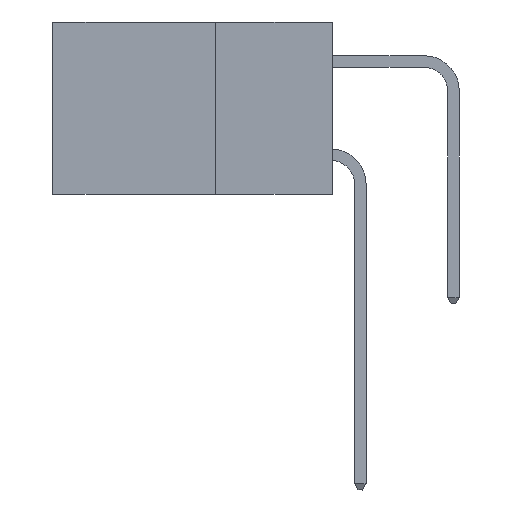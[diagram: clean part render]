
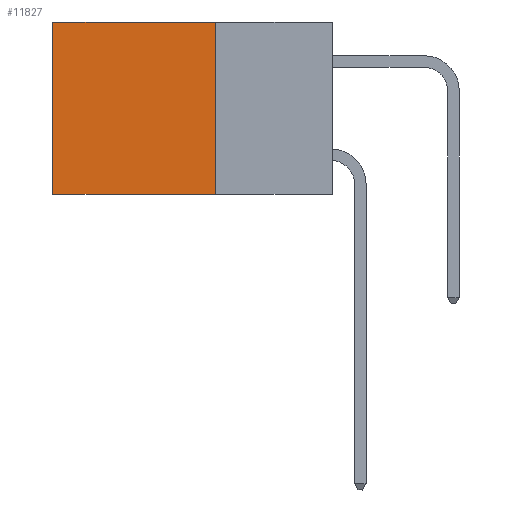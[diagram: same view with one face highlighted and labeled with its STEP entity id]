
A CAD part, left-side view. The second image highlights one B-rep face of the part: STEP entity #11827.
In plain terms, the highlighted planar face has unit normal (-1, 0, 0).
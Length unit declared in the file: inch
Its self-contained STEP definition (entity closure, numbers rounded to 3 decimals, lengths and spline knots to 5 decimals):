
#1057 = LINE ( 'NONE', #18911, #16242 ) ;
#1133 = CARTESIAN_POINT ( 'NONE',  ( 0.298, 0.6, -0.37 ) ) ;
#1225 = CARTESIAN_POINT ( 'NONE',  ( 0.298, 0.25, -0.37 ) ) ;
#1312 = CARTESIAN_POINT ( 'NONE',  ( 0.298, 0.25, 0. ) ) ;
#4506 = VECTOR ( 'NONE', #20226, 39.37008 ) ;
#4579 = VERTEX_POINT ( 'NONE', #21825 ) ;
#4762 = CARTESIAN_POINT ( 'NONE',  ( 0.298, 0.6, 0. ) ) ;
#5280 = VECTOR ( 'NONE', #11885, 39.37008 ) ;
#8067 = LINE ( 'NONE', #1225, #18073 ) ;
#8236 = DIRECTION ( 'NONE',  ( 0., 1., 0. ) ) ;
#8670 = EDGE_CURVE ( 'NONE', #22129, #4579, #19409, .T. ) ;
#9235 = ORIENTED_EDGE ( 'NONE', *, *, #16340, .F. ) ;
#9587 = CARTESIAN_POINT ( 'NONE',  ( 0.298, 0.25, 0. ) ) ;
#9649 = AXIS2_PLACEMENT_3D ( 'NONE', #19230, #20927, #10399 ) ;
#10399 = DIRECTION ( 'NONE',  ( 0., 0., -1. ) ) ;
#11432 = ORIENTED_EDGE ( 'NONE', *, *, #15530, .T. ) ;
#11457 = EDGE_LOOP ( 'NONE', ( #15982, #9235, #14515, #11432 ) ) ;
#11827 = ADVANCED_FACE ( 'NONE', ( #12452 ), #13889, .F. ) ;
#11861 = DIRECTION ( 'NONE',  ( 0., 0., -1. ) ) ;
#11885 = DIRECTION ( 'NONE',  ( 0., 0., -1. ) ) ;
#12452 = FACE_OUTER_BOUND ( 'NONE', #11457, .T. ) ;
#13808 = EDGE_CURVE ( 'NONE', #22680, #18393, #1057, .T. ) ;
#13889 = PLANE ( 'NONE',  #9649 ) ;
#14515 = ORIENTED_EDGE ( 'NONE', *, *, #8670, .F. ) ;
#15530 = EDGE_CURVE ( 'NONE', #22129, #22680, #18659, .T. ) ;
#15982 = ORIENTED_EDGE ( 'NONE', *, *, #13808, .T. ) ;
#16242 = VECTOR ( 'NONE', #11861, 39.37008 ) ;
#16340 = EDGE_CURVE ( 'NONE', #4579, #18393, #8067, .T. ) ;
#17671 = CARTESIAN_POINT ( 'NONE',  ( 0.298, 0.25, 0. ) ) ;
#18073 = VECTOR ( 'NONE', #8236, 39.37008 ) ;
#18393 = VERTEX_POINT ( 'NONE', #1133 ) ;
#18659 = LINE ( 'NONE', #9587, #4506 ) ;
#18911 = CARTESIAN_POINT ( 'NONE',  ( 0.298, 0.6, 0. ) ) ;
#19230 = CARTESIAN_POINT ( 'NONE',  ( 0.298, 0.25, 0. ) ) ;
#19409 = LINE ( 'NONE', #1312, #5280 ) ;
#20226 = DIRECTION ( 'NONE',  ( 0., 1., 0. ) ) ;
#20927 = DIRECTION ( 'NONE',  ( 1., 0., 0. ) ) ;
#21825 = CARTESIAN_POINT ( 'NONE',  ( 0.298, 0.25, -0.37 ) ) ;
#22129 = VERTEX_POINT ( 'NONE', #17671 ) ;
#22680 = VERTEX_POINT ( 'NONE', #4762 ) ;
